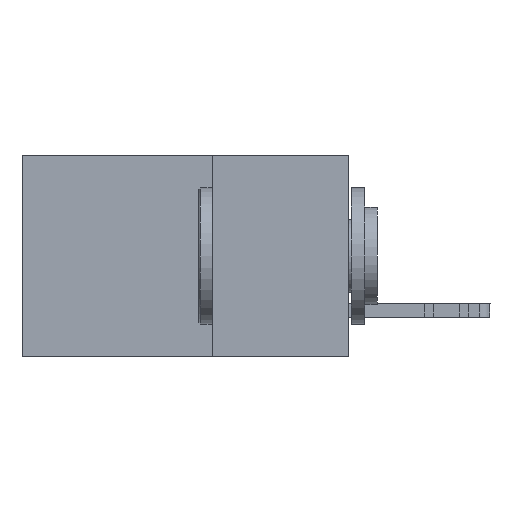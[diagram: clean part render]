
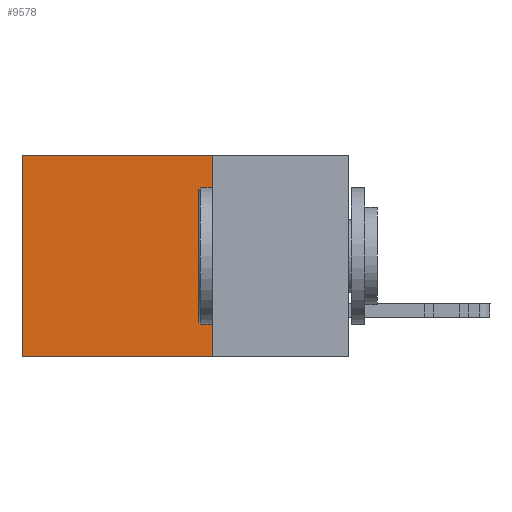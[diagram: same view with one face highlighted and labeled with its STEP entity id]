
A CAD part, left-side view. The second image highlights one B-rep face of the part: STEP entity #9578.
In plain terms, the highlighted planar face has unit normal (-1, 0, 0).
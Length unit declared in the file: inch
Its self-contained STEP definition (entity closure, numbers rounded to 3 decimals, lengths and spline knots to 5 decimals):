
#170 = VERTEX_POINT ( 'NONE', #19976 ) ;
#228 = DIRECTION ( 'NONE',  ( 0., 0., -1. ) ) ;
#568 = CARTESIAN_POINT ( 'NONE',  ( 0.298, 0.25, 0. ) ) ;
#2641 = DIRECTION ( 'NONE',  ( 1., 0., 0. ) ) ;
#3413 = EDGE_CURVE ( 'NONE', #8103, #6498, #28462, .T. ) ;
#3687 = LINE ( 'NONE', #568, #15262 ) ;
#4131 = DIRECTION ( 'NONE',  ( 0., 1., 0. ) ) ;
#4438 = EDGE_LOOP ( 'NONE', ( #10923, #11890, #24012, #19332 ) ) ;
#5069 = CARTESIAN_POINT ( 'NONE',  ( 0.298, 0.25, 0. ) ) ;
#5692 = EDGE_CURVE ( 'NONE', #170, #20633, #28573, .T. ) ;
#6498 = VERTEX_POINT ( 'NONE', #17441 ) ;
#6836 = EDGE_CURVE ( 'NONE', #6498, #20633, #16176, .T. ) ;
#8103 = VERTEX_POINT ( 'NONE', #14072 ) ;
#9036 = EDGE_CURVE ( 'NONE', #8103, #170, #3687, .T. ) ;
#9383 = VECTOR ( 'NONE', #20108, 39.37008 ) ;
#9578 = ADVANCED_FACE ( 'NONE', ( #24677 ), #9822, .F. ) ;
#9822 = PLANE ( 'NONE',  #19055 ) ;
#10923 = ORIENTED_EDGE ( 'NONE', *, *, #6836, .T. ) ;
#11890 = ORIENTED_EDGE ( 'NONE', *, *, #5692, .F. ) ;
#14072 = CARTESIAN_POINT ( 'NONE',  ( 0.298, 0.25, 0. ) ) ;
#14849 = CARTESIAN_POINT ( 'NONE',  ( 0.298, 0.25, 0. ) ) ;
#15262 = VECTOR ( 'NONE', #19082, 39.37008 ) ;
#15329 = CARTESIAN_POINT ( 'NONE',  ( 0.298, 0.6, -0.37 ) ) ;
#16176 = LINE ( 'NONE', #29485, #26683 ) ;
#17441 = CARTESIAN_POINT ( 'NONE',  ( 0.298, 0.6, 0. ) ) ;
#17458 = DIRECTION ( 'NONE',  ( 0., 0., -1. ) ) ;
#18678 = VECTOR ( 'NONE', #4131, 39.37008 ) ;
#19055 = AXIS2_PLACEMENT_3D ( 'NONE', #5069, #2641, #228 ) ;
#19082 = DIRECTION ( 'NONE',  ( 0., 0., -1. ) ) ;
#19332 = ORIENTED_EDGE ( 'NONE', *, *, #3413, .T. ) ;
#19976 = CARTESIAN_POINT ( 'NONE',  ( 0.298, 0.25, -0.37 ) ) ;
#20108 = DIRECTION ( 'NONE',  ( 0., 1., 0. ) ) ;
#20633 = VERTEX_POINT ( 'NONE', #15329 ) ;
#24012 = ORIENTED_EDGE ( 'NONE', *, *, #9036, .F. ) ;
#24677 = FACE_OUTER_BOUND ( 'NONE', #4438, .T. ) ;
#26683 = VECTOR ( 'NONE', #17458, 39.37008 ) ;
#27007 = CARTESIAN_POINT ( 'NONE',  ( 0.298, 0.25, -0.37 ) ) ;
#28462 = LINE ( 'NONE', #14849, #18678 ) ;
#28573 = LINE ( 'NONE', #27007, #9383 ) ;
#29485 = CARTESIAN_POINT ( 'NONE',  ( 0.298, 0.6, 0. ) ) ;
